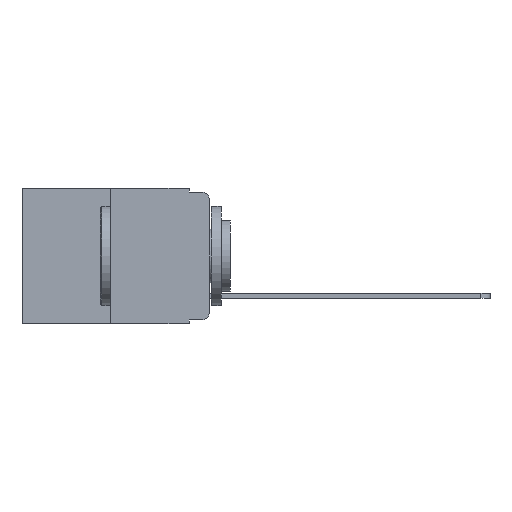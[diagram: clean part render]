
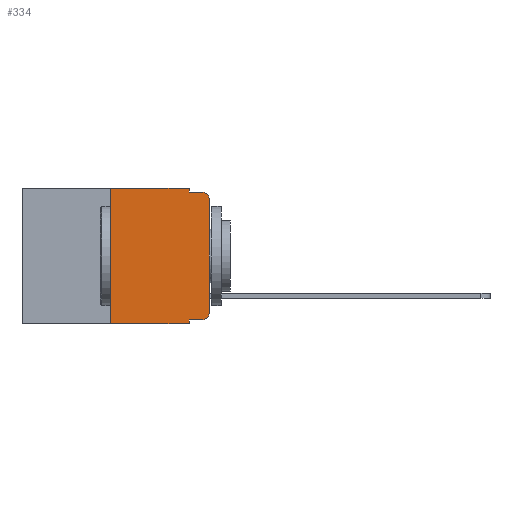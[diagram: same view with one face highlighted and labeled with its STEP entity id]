
A CAD part, left-side view. The second image highlights one B-rep face of the part: STEP entity #334.
In plain terms, the highlighted planar face has unit normal (-1, 0, 0).
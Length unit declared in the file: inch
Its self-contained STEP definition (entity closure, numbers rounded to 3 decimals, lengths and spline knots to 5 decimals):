
#252 = CARTESIAN_POINT ( 'NONE',  ( 0., 0.051, -0.333 ) ) ;
#324 = VECTOR ( 'NONE', #8929, 39.37008 ) ;
#334 = ADVANCED_FACE ( 'NONE', ( #6772 ), #4062, .F. ) ;
#581 = CARTESIAN_POINT ( 'NONE',  ( 0., 0.051, -0.01 ) ) ;
#679 = CARTESIAN_POINT ( 'NONE',  ( 0., 0.051, -0.333 ) ) ;
#704 = LINE ( 'NONE', #2491, #324 ) ;
#728 = ORIENTED_EDGE ( 'NONE', *, *, #9213, .F. ) ;
#735 = DIRECTION ( 'NONE',  ( 0., 0., -1. ) ) ;
#1013 = VERTEX_POINT ( 'NONE', #3283 ) ;
#1154 = CARTESIAN_POINT ( 'NONE',  ( 0., 0.25, -0.343 ) ) ;
#1824 = DIRECTION ( 'NONE',  ( 0., -1., 0. ) ) ;
#1925 = LINE ( 'NONE', #5389, #6334 ) ;
#2165 = CARTESIAN_POINT ( 'NONE',  ( 0., 0.473, -0.343 ) ) ;
#2181 = CIRCLE ( 'NONE', #4826, 0.02 ) ;
#2194 = LINE ( 'NONE', #2165, #4008 ) ;
#2491 = CARTESIAN_POINT ( 'NONE',  ( 0., 0., 0. ) ) ;
#2684 = VERTEX_POINT ( 'NONE', #9749 ) ;
#2811 = VERTEX_POINT ( 'NONE', #9519 ) ;
#3283 = CARTESIAN_POINT ( 'NONE',  ( 0., 0.051, 0. ) ) ;
#3546 = CARTESIAN_POINT ( 'NONE',  ( 0., 0.02, -0.03 ) ) ;
#3561 = VERTEX_POINT ( 'NONE', #8185 ) ;
#3839 = ORIENTED_EDGE ( 'NONE', *, *, #9142, .T. ) ;
#3849 = ORIENTED_EDGE ( 'NONE', *, *, #9193, .T. ) ;
#3888 = ORIENTED_EDGE ( 'NONE', *, *, #9194, .F. ) ;
#3902 = ORIENTED_EDGE ( 'NONE', *, *, #9207, .F. ) ;
#3914 = ORIENTED_EDGE ( 'NONE', *, *, #8546, .F. ) ;
#3929 = AXIS2_PLACEMENT_3D ( 'NONE', #3983, #8293, #4007 ) ;
#3937 = ORIENTED_EDGE ( 'NONE', *, *, #8917, .T. ) ;
#3947 = ORIENTED_EDGE ( 'NONE', *, *, #9224, .F. ) ;
#3964 = ORIENTED_EDGE ( 'NONE', *, *, #9226, .T. ) ;
#3967 = ORIENTED_EDGE ( 'NONE', *, *, #9238, .T. ) ;
#3983 = CARTESIAN_POINT ( 'NONE',  ( 0., 0.473, 0. ) ) ;
#3998 = LINE ( 'NONE', #7668, #8015 ) ;
#4007 = DIRECTION ( 'NONE',  ( 0., 0., -1. ) ) ;
#4008 = VECTOR ( 'NONE', #7278, 39.37008 ) ;
#4062 = PLANE ( 'NONE',  #3929 ) ;
#4291 = LINE ( 'NONE', #581, #9981 ) ;
#4453 = DIRECTION ( 'NONE',  ( 0., 0., -1. ) ) ;
#4826 = AXIS2_PLACEMENT_3D ( 'NONE', #3546, #9048, #4453 ) ;
#4878 = AXIS2_PLACEMENT_3D ( 'NONE', #10289, #6256, #735 ) ;
#5170 = EDGE_LOOP ( 'NONE', ( #3839, #3849, #3888, #3902, #3914, #728, #3937, #3947, #3964, #3967 ) ) ;
#5287 = VERTEX_POINT ( 'NONE', #9839 ) ;
#5389 = CARTESIAN_POINT ( 'NONE',  ( 0., 0.051, 0. ) ) ;
#5424 = CARTESIAN_POINT ( 'NONE',  ( 0., 0.051, 0. ) ) ;
#5486 = VECTOR ( 'NONE', #6530, 39.37008 ) ;
#5812 = VECTOR ( 'NONE', #1824, 39.37008 ) ;
#6053 = LINE ( 'NONE', #5424, #8457 ) ;
#6058 = VERTEX_POINT ( 'NONE', #252 ) ;
#6184 = DIRECTION ( 'NONE',  ( 0., 0., -1. ) ) ;
#6256 = DIRECTION ( 'NONE',  ( -1., 0., 0. ) ) ;
#6334 = VECTOR ( 'NONE', #6184, 39.37008 ) ;
#6530 = DIRECTION ( 'NONE',  ( 0., -1., 0. ) ) ;
#6772 = FACE_OUTER_BOUND ( 'NONE', #5170, .T. ) ;
#6880 = VERTEX_POINT ( 'NONE', #7361 ) ;
#7278 = DIRECTION ( 'NONE',  ( 0., -1., 0. ) ) ;
#7284 = VERTEX_POINT ( 'NONE', #1154 ) ;
#7346 = VERTEX_POINT ( 'NONE', #10173 ) ;
#7361 = CARTESIAN_POINT ( 'NONE',  ( 0., 0., -0.03 ) ) ;
#7626 = DIRECTION ( 'NONE',  ( 0., 0., -1. ) ) ;
#7668 = CARTESIAN_POINT ( 'NONE',  ( 0., 0.25, 0. ) ) ;
#8015 = VECTOR ( 'NONE', #8353, 39.37008 ) ;
#8185 = CARTESIAN_POINT ( 'NONE',  ( 0., 0., -0.313 ) ) ;
#8293 = DIRECTION ( 'NONE',  ( 1., 0., 0. ) ) ;
#8353 = DIRECTION ( 'NONE',  ( 0., 0., 1. ) ) ;
#8457 = VECTOR ( 'NONE', #7626, 39.37008 ) ;
#8546 = EDGE_CURVE ( 'NONE', #7346, #1013, #9579, .T. ) ;
#8917 = EDGE_CURVE ( 'NONE', #7284, #5287, #2194, .T. ) ;
#8929 = DIRECTION ( 'NONE',  ( 0., 0., 1. ) ) ;
#9009 = CARTESIAN_POINT ( 'NONE',  ( 0., 0.473, 0. ) ) ;
#9048 = DIRECTION ( 'NONE',  ( -1., 0., 0. ) ) ;
#9142 = EDGE_CURVE ( 'NONE', #3561, #6880, #704, .T. ) ;
#9193 = EDGE_CURVE ( 'NONE', #6880, #2684, #2181, .T. ) ;
#9194 = EDGE_CURVE ( 'NONE', #10219, #2684, #4291, .T. ) ;
#9207 = EDGE_CURVE ( 'NONE', #1013, #10219, #1925, .T. ) ;
#9213 = EDGE_CURVE ( 'NONE', #7284, #7346, #3998, .T. ) ;
#9224 = EDGE_CURVE ( 'NONE', #6058, #5287, #6053, .T. ) ;
#9226 = EDGE_CURVE ( 'NONE', #6058, #2811, #9656, .T. ) ;
#9238 = EDGE_CURVE ( 'NONE', #2811, #3561, #9821, .T. ) ;
#9519 = CARTESIAN_POINT ( 'NONE',  ( 0., 0.02, -0.333 ) ) ;
#9579 = LINE ( 'NONE', #9009, #5486 ) ;
#9656 = LINE ( 'NONE', #679, #5812 ) ;
#9749 = CARTESIAN_POINT ( 'NONE',  ( 0., 0.02, -0.01 ) ) ;
#9821 = CIRCLE ( 'NONE', #4878, 0.02 ) ;
#9839 = CARTESIAN_POINT ( 'NONE',  ( 0., 0.051, -0.343 ) ) ;
#9981 = VECTOR ( 'NONE', #10217, 39.37008 ) ;
#10168 = CARTESIAN_POINT ( 'NONE',  ( 0., 0.051, -0.01 ) ) ;
#10173 = CARTESIAN_POINT ( 'NONE',  ( 0., 0.25, 0. ) ) ;
#10217 = DIRECTION ( 'NONE',  ( 0., -1., 0. ) ) ;
#10219 = VERTEX_POINT ( 'NONE', #10168 ) ;
#10289 = CARTESIAN_POINT ( 'NONE',  ( 0., 0.02, -0.313 ) ) ;
